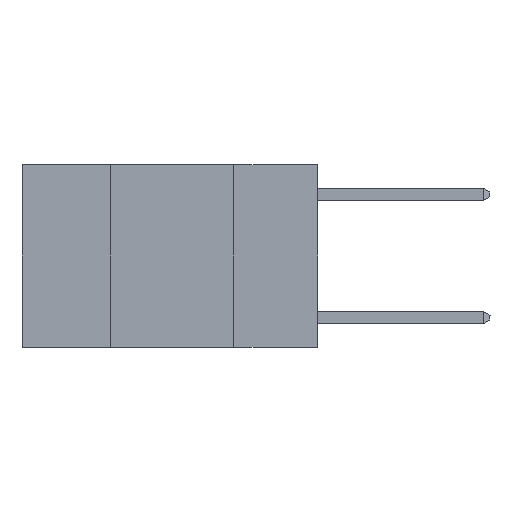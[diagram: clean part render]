
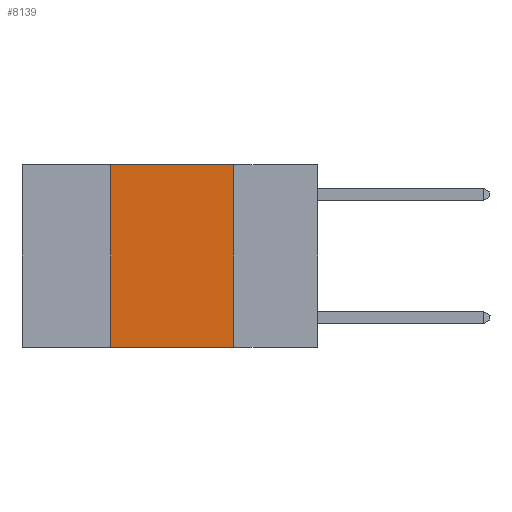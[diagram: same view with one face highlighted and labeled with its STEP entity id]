
A CAD part, left-side view. The second image highlights one B-rep face of the part: STEP entity #8139.
In plain terms, the highlighted planar face has unit normal (-1, 0, 0).
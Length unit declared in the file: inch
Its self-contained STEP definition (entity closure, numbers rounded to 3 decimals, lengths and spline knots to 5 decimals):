
#316 = EDGE_LOOP ( 'NONE', ( #7893, #7970, #8058, #8124 ) ) ;
#862 = CARTESIAN_POINT ( 'NONE',  ( 0., 0.17, 0. ) ) ;
#1133 = VERTEX_POINT ( 'NONE', #862 ) ;
#1738 = CARTESIAN_POINT ( 'NONE',  ( 0., 0.42, -0.37 ) ) ;
#1900 = DIRECTION ( 'NONE',  ( 0., 0., 1. ) ) ;
#2253 = DIRECTION ( 'NONE',  ( 0., -1., 0. ) ) ;
#2353 = EDGE_CURVE ( 'NONE', #9242, #5817, #10332, .T. ) ;
#2637 = VECTOR ( 'NONE', #1900, 39.37008 ) ;
#3751 = CARTESIAN_POINT ( 'NONE',  ( 0., 0.6, 0. ) ) ;
#4037 = FACE_OUTER_BOUND ( 'NONE', #316, .T. ) ;
#4088 = EDGE_CURVE ( 'NONE', #1133, #5817, #9348, .T. ) ;
#4287 = VECTOR ( 'NONE', #4841, 39.37008 ) ;
#4586 = CARTESIAN_POINT ( 'NONE',  ( 0., 0.17, -0.37 ) ) ;
#4841 = DIRECTION ( 'NONE',  ( 0., -1., 0. ) ) ;
#5219 = DIRECTION ( 'NONE',  ( 1., 0., 0. ) ) ;
#5817 = VERTEX_POINT ( 'NONE', #4586 ) ;
#6433 = VERTEX_POINT ( 'NONE', #10701 ) ;
#6869 = CARTESIAN_POINT ( 'NONE',  ( 0., 0.17, 0. ) ) ;
#7375 = VECTOR ( 'NONE', #2253, 39.37008 ) ;
#7893 = ORIENTED_EDGE ( 'NONE', *, *, #4088, .F. ) ;
#7970 = ORIENTED_EDGE ( 'NONE', *, *, #13435, .F. ) ;
#8058 = ORIENTED_EDGE ( 'NONE', *, *, #9369, .F. ) ;
#8124 = ORIENTED_EDGE ( 'NONE', *, *, #2353, .T. ) ;
#8139 = ADVANCED_FACE ( 'NONE', ( #4037 ), #10749, .F. ) ;
#8681 = VECTOR ( 'NONE', #12299, 39.37008 ) ;
#9242 = VERTEX_POINT ( 'NONE', #1738 ) ;
#9348 = LINE ( 'NONE', #6869, #8681 ) ;
#9369 = EDGE_CURVE ( 'NONE', #9242, #6433, #11746, .T. ) ;
#9948 = CARTESIAN_POINT ( 'NONE',  ( 0., 0.6, -0.37 ) ) ;
#10194 = LINE ( 'NONE', #3751, #4287 ) ;
#10332 = LINE ( 'NONE', #9948, #7375 ) ;
#10701 = CARTESIAN_POINT ( 'NONE',  ( 0., 0.42, 0. ) ) ;
#10749 = PLANE ( 'NONE',  #11117 ) ;
#10775 = CARTESIAN_POINT ( 'NONE',  ( 0., 0.42, 0. ) ) ;
#11117 = AXIS2_PLACEMENT_3D ( 'NONE', #11814, #5219, #12860 ) ;
#11746 = LINE ( 'NONE', #10775, #2637 ) ;
#11814 = CARTESIAN_POINT ( 'NONE',  ( 0., 0.6, 0. ) ) ;
#12299 = DIRECTION ( 'NONE',  ( 0., 0., -1. ) ) ;
#12860 = DIRECTION ( 'NONE',  ( 0., 0., -1. ) ) ;
#13435 = EDGE_CURVE ( 'NONE', #6433, #1133, #10194, .T. ) ;
